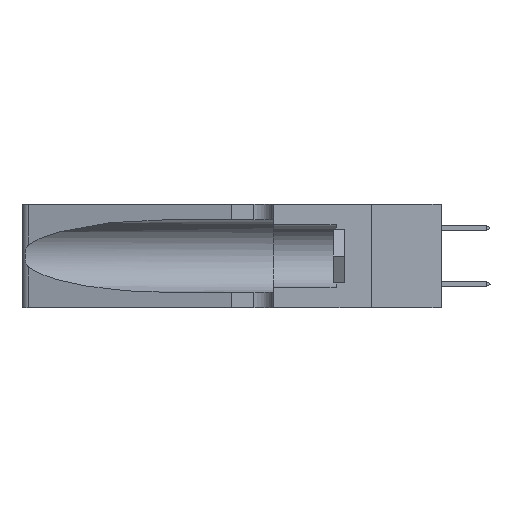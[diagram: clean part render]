
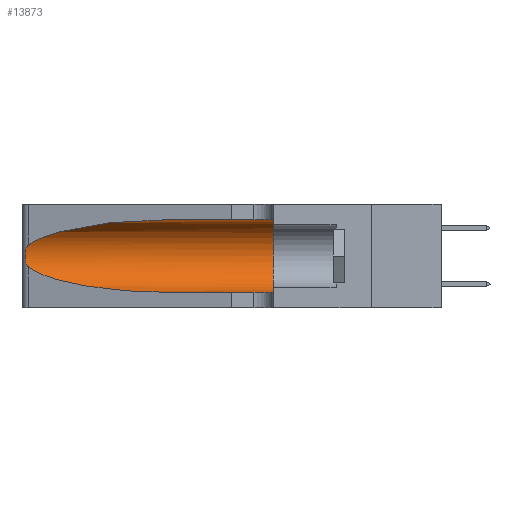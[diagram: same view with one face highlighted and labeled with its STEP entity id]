
A CAD part, left-side view. The second image highlights one B-rep face of the part: STEP entity #13873.
In plain terms, the highlighted cylindrical face has radius 3.308 mm (diameter 6.617 mm), a partial arc.
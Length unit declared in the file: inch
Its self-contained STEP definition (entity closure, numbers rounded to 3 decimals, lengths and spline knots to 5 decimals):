
#1640 = VERTEX_POINT ( 'NONE', #21059 ) ;
#2025 = LINE ( 'NONE', #29436, #19346 ) ;
#2289 = EDGE_CURVE ( 'NONE', #6141, #4651, #19125, .T. ) ;
#2363 = CARTESIAN_POINT ( 'NONE',  ( 0.25789, 1.23486, 0.15765 ) ) ;
#3100 = CYLINDRICAL_SURFACE ( 'NONE', #13125, 0.13025 ) ;
#3309 = ORIENTED_EDGE ( 'NONE', *, *, #21500, .F. ) ;
#3474 = CARTESIAN_POINT ( 'NONE',  ( 0.1305, 0.35, 0.185 ) ) ;
#3857 = FACE_OUTER_BOUND ( 'NONE', #29934, .T. ) ;
#4281 = EDGE_CURVE ( 'NONE', #4651, #25619, #27882, .T. ) ;
#4387 = DIRECTION ( 'NONE',  ( 0., 0., -1. ) ) ;
#4651 = VERTEX_POINT ( 'NONE', #29058 ) ;
#4803 = CARTESIAN_POINT ( 'NONE',  ( 0.25555, 1.22993, 0.14849 ) ) ;
#4855 = CARTESIAN_POINT ( 'NONE',  ( 0.25487, 1.22718, 0.14631 ) ) ;
#5899 = DIRECTION ( 'NONE',  ( 0., 0., 1. ) ) ;
#5955 = VECTOR ( 'NONE', #23100, 39.37008 ) ;
#6141 = VERTEX_POINT ( 'NONE', #25322 ) ;
#7246 = CARTESIAN_POINT ( 'NONE',  ( 0.2373, 1.15595, 0.08982 ) ) ;
#8026 = EDGE_CURVE ( 'NONE', #11124, #6141, #11116, .T. ) ;
#8536 = AXIS2_PLACEMENT_3D ( 'NONE', #3474, #19871, #5899 ) ;
#9072 = DIRECTION ( 'NONE',  ( 0., -1., 0. ) ) ;
#9478 = CARTESIAN_POINT ( 'NONE',  ( 0.25787, 1.23484, 0.2124 ) ) ;
#10677 = ORIENTED_EDGE ( 'NONE', *, *, #17289, .T. ) ;
#10790 = CARTESIAN_POINT ( 'NONE',  ( 0.18966, 0.96281, 0.31525 ) ) ;
#11116 =( BOUNDED_CURVE ( )  B_SPLINE_CURVE ( 3, ( #24576, #10790, #26811, #13170 ),
 .UNSPECIFIED., .F., .F. ) 
 B_SPLINE_CURVE_WITH_KNOTS ( ( 4, 4 ),
 ( 1.5708, 2.84003 ),
 .UNSPECIFIED. ) 
 CURVE ( )  GEOMETRIC_REPRESENTATION_ITEM ( )  RATIONAL_B_SPLINE_CURVE ( ( 1., 0.87, 0.87, 1. ) ) 
 REPRESENTATION_ITEM ( '' )  );
#11124 = VERTEX_POINT ( 'NONE', #22735 ) ;
#11543 = CARTESIAN_POINT ( 'NONE',  ( 0.1305, 1.61858, 0.31525 ) ) ;
#11856 = CARTESIAN_POINT ( 'NONE',  ( 0.26018, 1.23835, 0.19895 ) ) ;
#12009 = CARTESIAN_POINT ( 'NONE',  ( 0.1305, 0.72297, 0.05475 ) ) ;
#12294 = ORIENTED_EDGE ( 'NONE', *, *, #2289, .T. ) ;
#12640 = ORIENTED_EDGE ( 'NONE', *, *, #4281, .T. ) ;
#13125 = AXIS2_PLACEMENT_3D ( 'NONE', #27401, #9072, #4387 ) ;
#13170 = CARTESIAN_POINT ( 'NONE',  ( 0.25487, 1.22718, 0.22369 ) ) ;
#13873 = ADVANCED_FACE ( 'NONE', ( #3857 ), #3100, .F. ) ;
#14201 = CARTESIAN_POINT ( 'NONE',  ( 0.26075, 1.23896, 0.178 ) ) ;
#16409 = CARTESIAN_POINT ( 'NONE',  ( 0.25555, 1.22994, 0.2215 ) ) ;
#16468 = VERTEX_POINT ( 'NONE', #29586 ) ;
#16514 = CARTESIAN_POINT ( 'NONE',  ( 0.25856, 1.23593, 0.16098 ) ) ;
#17234 = ORIENTED_EDGE ( 'NONE', *, *, #23568, .F. ) ;
#17289 = EDGE_CURVE ( 'NONE', #25619, #16468, #2025, .T. ) ;
#18288 = DIRECTION ( 'NONE',  ( 0., -1., 0. ) ) ;
#18846 = CARTESIAN_POINT ( 'NONE',  ( 0.25639, 1.23186, 0.15144 ) ) ;
#19125 = B_SPLINE_CURVE_WITH_KNOTS ( 'NONE', 3,
 ( #23300, #16409, #29902, #9478, #25556, #11856, #27773, #14201, #30000, #16514, #2363, #18846, #4803, #21117 ),
 .UNSPECIFIED., .F., .F.,
 ( 4, 2, 2, 2, 2, 2, 4 ),
 ( 0., 0.00027, 0.00053, 0.00107, 0.0016, 0.00187, 0.00214 ),
 .UNSPECIFIED. ) ;
#19346 = VECTOR ( 'NONE', #18288, 39.37008 ) ;
#19871 = DIRECTION ( 'NONE',  ( 0., 1., 0. ) ) ;
#21059 = CARTESIAN_POINT ( 'NONE',  ( 0.1305, 0.35, 0.31525 ) ) ;
#21117 = CARTESIAN_POINT ( 'NONE',  ( 0.25487, 1.22718, 0.14631 ) ) ;
#21500 = EDGE_CURVE ( 'NONE', #1640, #16468, #22063, .T. ) ;
#22063 = CIRCLE ( 'NONE', #8536, 0.13025 ) ;
#22735 = CARTESIAN_POINT ( 'NONE',  ( 0.1305, 0.72297, 0.31525 ) ) ;
#23100 = DIRECTION ( 'NONE',  ( 0., -1., 0. ) ) ;
#23300 = CARTESIAN_POINT ( 'NONE',  ( 0.25487, 1.22718, 0.22369 ) ) ;
#23568 = EDGE_CURVE ( 'NONE', #11124, #1640, #24438, .T. ) ;
#24438 = LINE ( 'NONE', #11543, #5955 ) ;
#24576 = CARTESIAN_POINT ( 'NONE',  ( 0.1305, 0.72297, 0.31525 ) ) ;
#25322 = CARTESIAN_POINT ( 'NONE',  ( 0.25487, 1.22718, 0.22369 ) ) ;
#25556 = CARTESIAN_POINT ( 'NONE',  ( 0.25854, 1.2359, 0.20912 ) ) ;
#25619 = VERTEX_POINT ( 'NONE', #29711 ) ;
#25705 = CARTESIAN_POINT ( 'NONE',  ( 0.18966, 0.96281, 0.05475 ) ) ;
#26811 = CARTESIAN_POINT ( 'NONE',  ( 0.2373, 1.15595, 0.28018 ) ) ;
#27401 = CARTESIAN_POINT ( 'NONE',  ( 0.1305, 1.61858, 0.185 ) ) ;
#27773 = CARTESIAN_POINT ( 'NONE',  ( 0.26075, 1.23896, 0.19203 ) ) ;
#27882 =( BOUNDED_CURVE ( )  B_SPLINE_CURVE ( 3, ( #4855, #7246, #25705, #12009 ),
 .UNSPECIFIED., .F., .F. ) 
 B_SPLINE_CURVE_WITH_KNOTS ( ( 4, 4 ),
 ( 3.44316, 4.71239 ),
 .UNSPECIFIED. ) 
 CURVE ( )  GEOMETRIC_REPRESENTATION_ITEM ( )  RATIONAL_B_SPLINE_CURVE ( ( 1., 0.87, 0.87, 1. ) ) 
 REPRESENTATION_ITEM ( '' )  );
#28712 = ORIENTED_EDGE ( 'NONE', *, *, #8026, .T. ) ;
#29058 = CARTESIAN_POINT ( 'NONE',  ( 0.25487, 1.22718, 0.14631 ) ) ;
#29436 = CARTESIAN_POINT ( 'NONE',  ( 0.1305, 1.61858, 0.05475 ) ) ;
#29586 = CARTESIAN_POINT ( 'NONE',  ( 0.1305, 0.35, 0.05475 ) ) ;
#29711 = CARTESIAN_POINT ( 'NONE',  ( 0.1305, 0.72297, 0.05475 ) ) ;
#29902 = CARTESIAN_POINT ( 'NONE',  ( 0.25639, 1.23184, 0.21858 ) ) ;
#29934 = EDGE_LOOP ( 'NONE', ( #28712, #12294, #12640, #10677, #3309, #17234 ) ) ;
#30000 = CARTESIAN_POINT ( 'NONE',  ( 0.26017, 1.23833, 0.17102 ) ) ;
